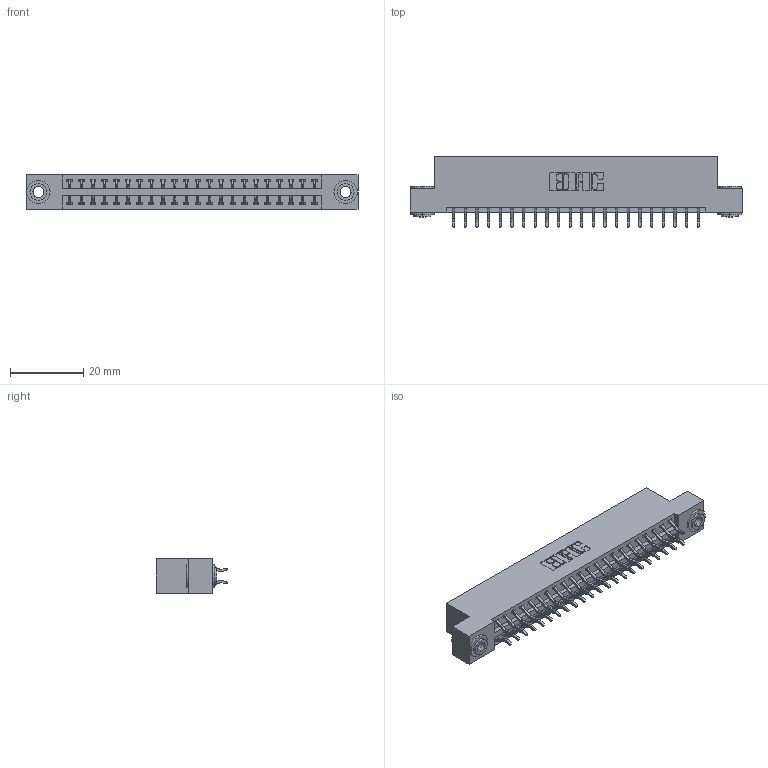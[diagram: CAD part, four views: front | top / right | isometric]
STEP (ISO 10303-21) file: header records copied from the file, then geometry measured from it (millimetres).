
FILE_DESCRIPTION (( 'STEP AP203' ), '1' );
FILE_NAME ('396-044-556-203.STEP', '2018-09-07T04:53:41', ( '' ), ( '' ), 'SwSTEP 2.0', 'SolidWorks 2016', '' );
FILE_SCHEMA (( 'CONFIG_CONTROL_DESIGN' ));
Length unit declared in the file: inch
Products named in the file (4): 346 Part_Flush Mounting Lugs - 0.156 Dia-TH; 345-292-001_556 Tail; 345-250-002_345-250-002-102; 396-044-556-203
Assembly tree (47 placements, depth 2):
  396-044-556-203
    346 Part_Flush Mounting Lugs - 0.156 Dia-TH
    345-292-001_556 Tail  x44
    345-250-002_345-250-002-102  x2
Bounding box: 90.42 x 19.57 x 9.4 mm (x, y, z)
Volume: 8679.8 mm3; surface area: 11789.9 mm2
Topology: 47 solids, 47 shells, 2712 faces, 8017 edges, 5282 vertices
Faces by surface type: plane 1802, cylinder 902, cone 8
Entity records: 17920 total; most frequent: CARTESIAN_POINT 2971, ORIENTED_EDGE 2886, DIRECTION 2689, EDGE_CURVE 1443, LINE 1191, VECTOR 1191, VERTEX_POINT 958, AXIS2_PLACEMENT_3D 749
